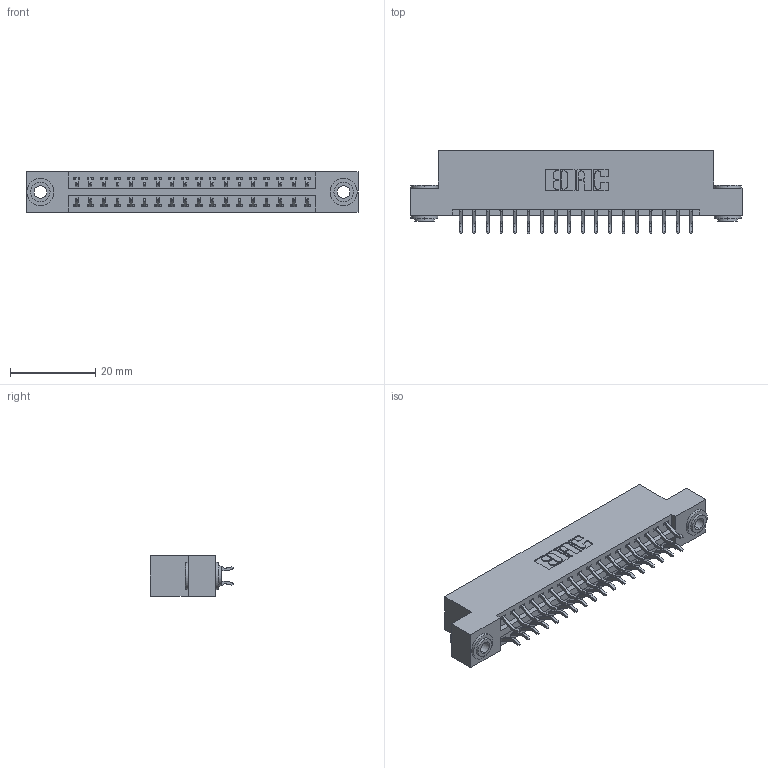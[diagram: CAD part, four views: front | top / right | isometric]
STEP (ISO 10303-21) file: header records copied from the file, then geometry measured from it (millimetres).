
FILE_DESCRIPTION (( 'STEP AP203' ), '1' );
FILE_NAME ('396-036-556-203.STEP', '2018-09-06T04:57:05', ( '' ), ( '' ), 'SwSTEP 2.0', 'SolidWorks 2016', '' );
FILE_SCHEMA (( 'CONFIG_CONTROL_DESIGN' ));
Length unit declared in the file: inch
Products named in the file (4): 396-036-556-203; 346 Part_Flush Mounting Lugs - 0.156 Dia-TH; 345-292-001_556 Tail; 345-250-002_345-250-002-102
Assembly tree (39 placements, depth 2):
  396-036-556-203
    346 Part_Flush Mounting Lugs - 0.156 Dia-TH
    345-292-001_556 Tail  x36
    345-250-002_345-250-002-102  x2
Bounding box: 77.72 x 19.57 x 9.4 mm (x, y, z)
Volume: 7410.6 mm3; surface area: 9989.9 mm2
Topology: 39 solids, 39 shells, 2248 faces, 6633 edges, 4370 vertices
Faces by surface type: plane 1490, cylinder 750, cone 8
Entity records: 15848 total; most frequent: CARTESIAN_POINT 2635, ORIENTED_EDGE 2550, DIRECTION 2393, EDGE_CURVE 1275, VECTOR 1039, LINE 1039, VERTEX_POINT 846, AXIS2_PLACEMENT_3D 677
